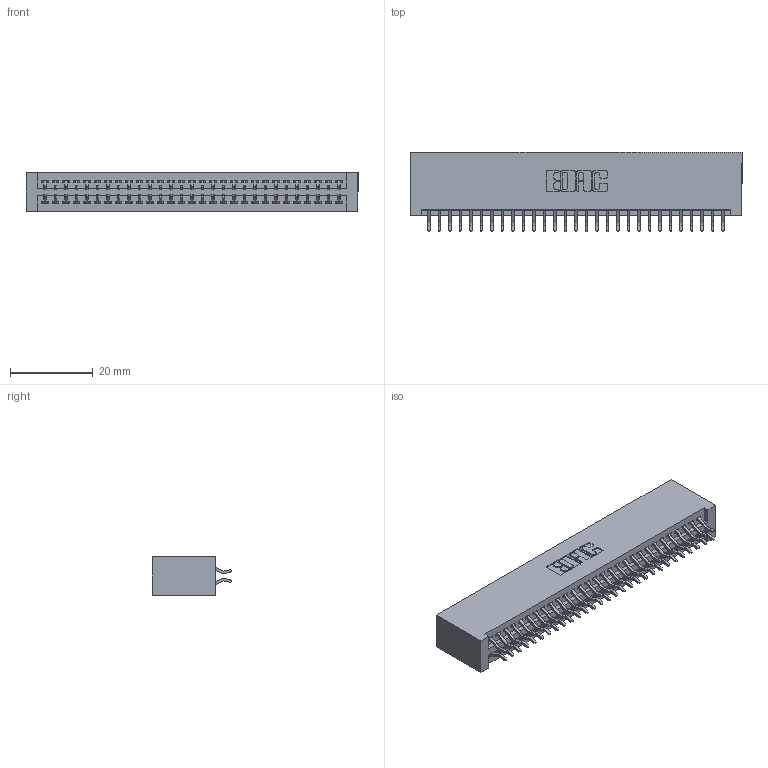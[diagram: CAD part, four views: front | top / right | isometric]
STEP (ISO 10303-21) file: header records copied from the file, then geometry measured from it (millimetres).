
FILE_DESCRIPTION (( 'STEP AP203' ), '1' );
FILE_NAME ('345-058-556-201.STEP', '2018-09-26T16:30:59', ( '' ), ( '' ), 'SwSTEP 2.0', 'SolidWorks 2016', '' );
FILE_SCHEMA (( 'CONFIG_CONTROL_DESIGN' ));
Length unit declared in the file: inch
Products named in the file (3): 345 Part_No Mounting Lugs; 345-058-556-201; 345-292-001_556 Tail
Assembly tree (59 placements, depth 2):
  345-058-556-201
    345 Part_No Mounting Lugs
    345-292-001_556 Tail  x58
Bounding box: 80.26 x 19.24 x 9.4 mm (x, y, z)
Volume: 8289.9 mm3; surface area: 12254.5 mm2
Topology: 59 solids, 59 shells, 3366 faces, 10003 edges, 6590 vertices
Faces by surface type: plane 2222, cylinder 1144
Entity records: 24447 total; most frequent: CARTESIAN_POINT 4124, ORIENTED_EDGE 4046, DIRECTION 3635, EDGE_CURVE 2023, VECTOR 1775, LINE 1775, VERTEX_POINT 1346, AXIS2_PLACEMENT_3D 930
